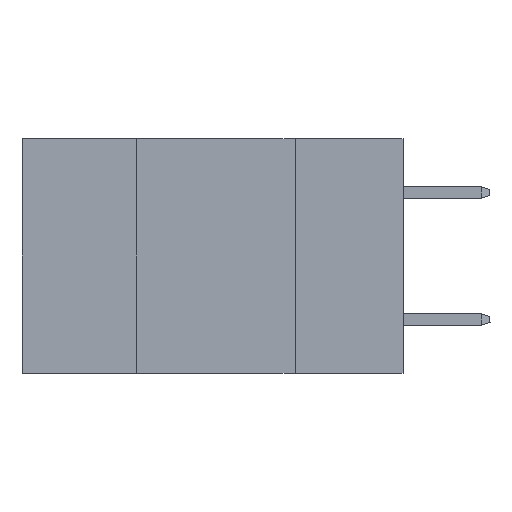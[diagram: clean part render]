
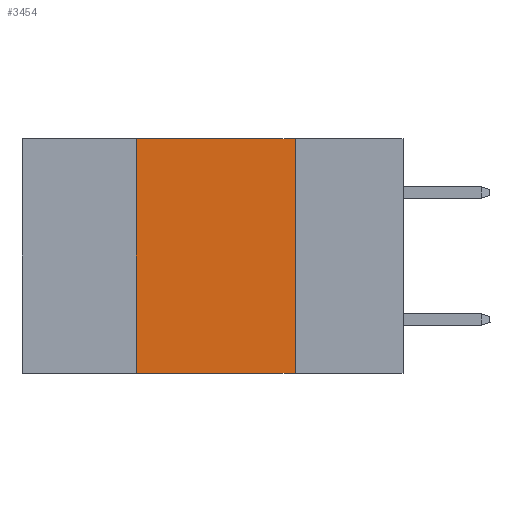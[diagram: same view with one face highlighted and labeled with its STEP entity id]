
A CAD part, left-side view. The second image highlights one B-rep face of the part: STEP entity #3454.
In plain terms, the highlighted planar face has unit normal (-1, 0, 0).
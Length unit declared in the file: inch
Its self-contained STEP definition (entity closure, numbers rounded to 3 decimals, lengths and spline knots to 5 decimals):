
#389 = VERTEX_POINT ( 'NONE', #9971 ) ;
#814 = VECTOR ( 'NONE', #1363, 39.37008 ) ;
#1265 = CARTESIAN_POINT ( 'NONE',  ( 0., 0.42, 0. ) ) ;
#1363 = DIRECTION ( 'NONE',  ( 0., 0., -1. ) ) ;
#2039 = VECTOR ( 'NONE', #5446, 39.37008 ) ;
#2801 = CARTESIAN_POINT ( 'NONE',  ( 0., 0.17, 0. ) ) ;
#3246 = EDGE_LOOP ( 'NONE', ( #3540, #14484, #7517, #5387 ) ) ;
#3454 = ADVANCED_FACE ( 'NONE', ( #4033 ), #6978, .F. ) ;
#3540 = ORIENTED_EDGE ( 'NONE', *, *, #15828, .F. ) ;
#3949 = CARTESIAN_POINT ( 'NONE',  ( 0., 0.6, 0. ) ) ;
#4033 = FACE_OUTER_BOUND ( 'NONE', #3246, .T. ) ;
#5290 = EDGE_CURVE ( 'NONE', #15212, #17532, #7655, .T. ) ;
#5359 = CARTESIAN_POINT ( 'NONE',  ( 0., 0.17, -0.37 ) ) ;
#5387 = ORIENTED_EDGE ( 'NONE', *, *, #9069, .T. ) ;
#5446 = DIRECTION ( 'NONE',  ( 0., 0., 1. ) ) ;
#6547 = AXIS2_PLACEMENT_3D ( 'NONE', #3949, #18558, #11270 ) ;
#6978 = PLANE ( 'NONE',  #6547 ) ;
#7517 = ORIENTED_EDGE ( 'NONE', *, *, #17471, .F. ) ;
#7655 = LINE ( 'NONE', #15002, #10579 ) ;
#8389 = CARTESIAN_POINT ( 'NONE',  ( 0., 0.17, 0. ) ) ;
#8881 = LINE ( 'NONE', #11555, #16592 ) ;
#9069 = EDGE_CURVE ( 'NONE', #389, #17519, #8881, .T. ) ;
#9971 = CARTESIAN_POINT ( 'NONE',  ( 0., 0.42, -0.37 ) ) ;
#10579 = VECTOR ( 'NONE', #17759, 39.37008 ) ;
#11270 = DIRECTION ( 'NONE',  ( 0., 0., -1. ) ) ;
#11555 = CARTESIAN_POINT ( 'NONE',  ( 0., 0.6, -0.37 ) ) ;
#14484 = ORIENTED_EDGE ( 'NONE', *, *, #5290, .F. ) ;
#14513 = DIRECTION ( 'NONE',  ( 0., -1., 0. ) ) ;
#15002 = CARTESIAN_POINT ( 'NONE',  ( 0., 0.6, 0. ) ) ;
#15212 = VERTEX_POINT ( 'NONE', #15756 ) ;
#15734 = LINE ( 'NONE', #1265, #2039 ) ;
#15756 = CARTESIAN_POINT ( 'NONE',  ( 0., 0.42, 0. ) ) ;
#15828 = EDGE_CURVE ( 'NONE', #17532, #17519, #18663, .T. ) ;
#16592 = VECTOR ( 'NONE', #14513, 39.37008 ) ;
#17471 = EDGE_CURVE ( 'NONE', #389, #15212, #15734, .T. ) ;
#17519 = VERTEX_POINT ( 'NONE', #5359 ) ;
#17532 = VERTEX_POINT ( 'NONE', #8389 ) ;
#17759 = DIRECTION ( 'NONE',  ( 0., -1., 0. ) ) ;
#18558 = DIRECTION ( 'NONE',  ( 1., 0., 0. ) ) ;
#18663 = LINE ( 'NONE', #2801, #814 ) ;
